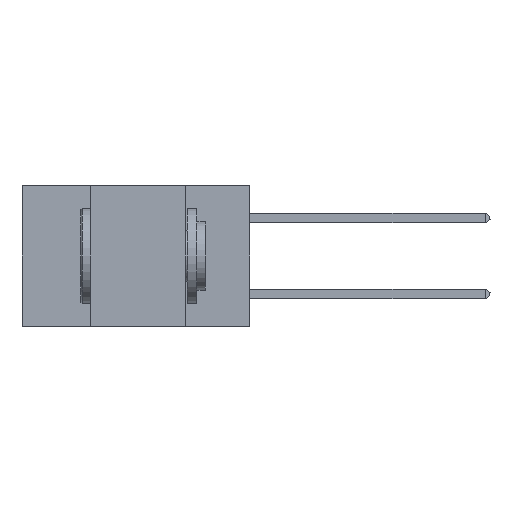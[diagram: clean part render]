
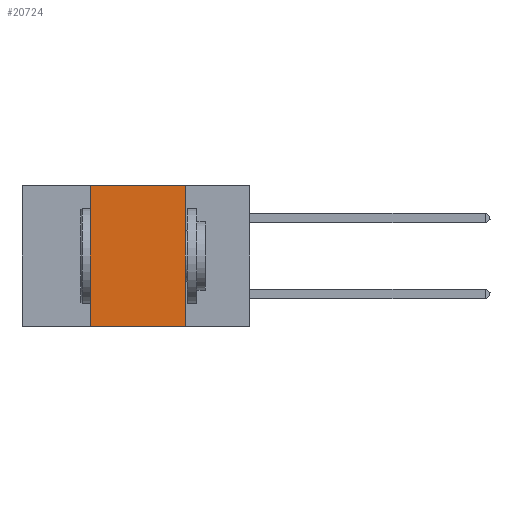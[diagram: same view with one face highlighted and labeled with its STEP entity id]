
A CAD part, left-side view. The second image highlights one B-rep face of the part: STEP entity #20724.
In plain terms, the highlighted planar face has unit normal (-1, 0, 0).
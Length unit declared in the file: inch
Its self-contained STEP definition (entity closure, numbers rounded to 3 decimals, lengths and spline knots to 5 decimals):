
#766 = EDGE_CURVE ( 'NONE', #32728, #21321, #14750, .T. ) ;
#3495 = VECTOR ( 'NONE', #20455, 39.37008 ) ;
#3738 = PLANE ( 'NONE',  #25750 ) ;
#5636 = CARTESIAN_POINT ( 'NONE',  ( 0., 0.6, 0. ) ) ;
#6097 = CARTESIAN_POINT ( 'NONE',  ( 0., 0.42, 0. ) ) ;
#6423 = DIRECTION ( 'NONE',  ( 0., 0., -1. ) ) ;
#6924 = DIRECTION ( 'NONE',  ( 1., 0., 0. ) ) ;
#7497 = EDGE_LOOP ( 'NONE', ( #31100, #17514, #34426, #20728 ) ) ;
#8747 = CARTESIAN_POINT ( 'NONE',  ( 0., 0.17, -0.37 ) ) ;
#9538 = LINE ( 'NONE', #37221, #26796 ) ;
#10215 = LINE ( 'NONE', #24068, #30822 ) ;
#12340 = EDGE_CURVE ( 'NONE', #32547, #21321, #10215, .T. ) ;
#13181 = CARTESIAN_POINT ( 'NONE',  ( 0., 0.6, 0. ) ) ;
#14750 = LINE ( 'NONE', #31579, #23838 ) ;
#16385 = CARTESIAN_POINT ( 'NONE',  ( 0., 0.17, 0. ) ) ;
#17514 = ORIENTED_EDGE ( 'NONE', *, *, #23570, .F. ) ;
#18146 = VERTEX_POINT ( 'NONE', #6097 ) ;
#19054 = DIRECTION ( 'NONE',  ( 0., 0., 1. ) ) ;
#20455 = DIRECTION ( 'NONE',  ( 0., -1., 0. ) ) ;
#20724 = ADVANCED_FACE ( 'NONE', ( #28075 ), #3738, .F. ) ;
#20728 = ORIENTED_EDGE ( 'NONE', *, *, #766, .T. ) ;
#21321 = VERTEX_POINT ( 'NONE', #8747 ) ;
#23570 = EDGE_CURVE ( 'NONE', #18146, #32547, #37010, .T. ) ;
#23838 = VECTOR ( 'NONE', #28294, 39.37008 ) ;
#24068 = CARTESIAN_POINT ( 'NONE',  ( 0., 0.17, 0. ) ) ;
#24999 = DIRECTION ( 'NONE',  ( 0., 0., -1. ) ) ;
#25750 = AXIS2_PLACEMENT_3D ( 'NONE', #13181, #6924, #24999 ) ;
#25802 = CARTESIAN_POINT ( 'NONE',  ( 0., 0.42, -0.37 ) ) ;
#26796 = VECTOR ( 'NONE', #19054, 39.37008 ) ;
#28075 = FACE_OUTER_BOUND ( 'NONE', #7497, .T. ) ;
#28294 = DIRECTION ( 'NONE',  ( 0., -1., 0. ) ) ;
#30822 = VECTOR ( 'NONE', #6423, 39.37008 ) ;
#31100 = ORIENTED_EDGE ( 'NONE', *, *, #12340, .F. ) ;
#31579 = CARTESIAN_POINT ( 'NONE',  ( 0., 0.6, -0.37 ) ) ;
#31656 = EDGE_CURVE ( 'NONE', #32728, #18146, #9538, .T. ) ;
#32547 = VERTEX_POINT ( 'NONE', #16385 ) ;
#32728 = VERTEX_POINT ( 'NONE', #25802 ) ;
#34426 = ORIENTED_EDGE ( 'NONE', *, *, #31656, .F. ) ;
#37010 = LINE ( 'NONE', #5636, #3495 ) ;
#37221 = CARTESIAN_POINT ( 'NONE',  ( 0., 0.42, 0. ) ) ;
